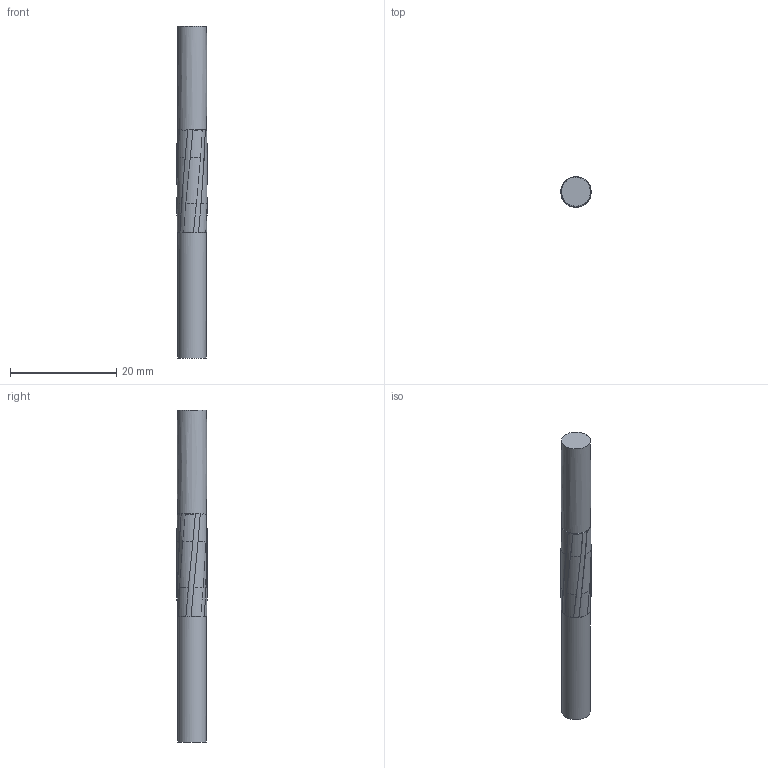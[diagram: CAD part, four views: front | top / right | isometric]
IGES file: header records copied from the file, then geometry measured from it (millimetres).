
Global section: file name: (5.56mm,223rem) rifling button; native system: Autodesk Inventor 2019; preprocessor: unknown; author: user; date: 20200917.141525; units: millimetre
Bounding box: 5.75 x 5.74 x 62.55 mm (x, y, z)
Volume: 1483 mm3; surface area: 1155.8 mm2
Topology: 1 solids, 1 shells, 48 faces, 141 edges, 95 vertices
Faces by surface type: bspline 48
